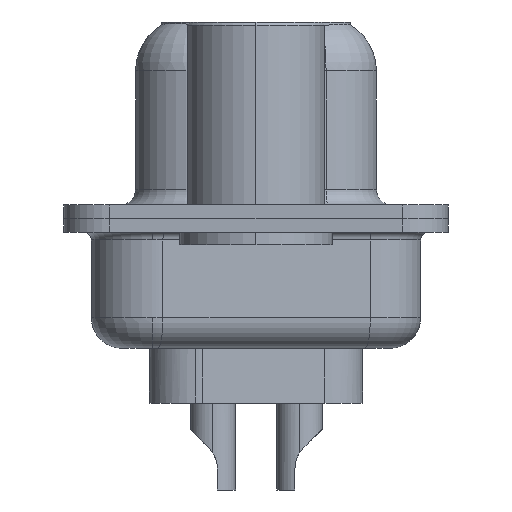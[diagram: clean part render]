
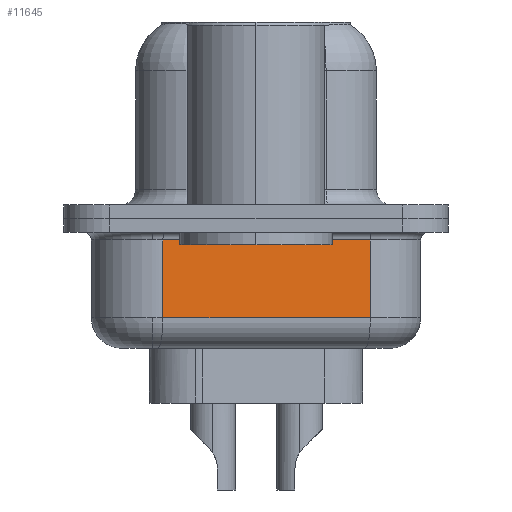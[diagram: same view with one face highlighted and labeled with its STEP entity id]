
A CAD part, left-side view. The second image highlights one B-rep face of the part: STEP entity #11645.
In plain terms, the highlighted planar face has unit normal (-0.985, -0.174, 0).
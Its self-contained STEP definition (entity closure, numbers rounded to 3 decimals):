
#163 = VECTOR ( 'NONE', #10738, 1000. ) ;
#1289 = AXIS2_PLACEMENT_3D ( 'NONE', #15558, #20677, #1568 ) ;
#1568 = DIRECTION ( 'NONE',  ( -0.174, 0.985, 0. ) ) ;
#2050 = DIRECTION ( 'NONE',  ( 0.174, -0.985, 0. ) ) ;
#2419 = EDGE_LOOP ( 'NONE', ( #8720, #7108, #7721, #17372 ) ) ;
#3175 = VERTEX_POINT ( 'NONE', #18210 ) ;
#3624 = DIRECTION ( 'NONE',  ( -0.174, 0.985, 0. ) ) ;
#3971 = CARTESIAN_POINT ( 'NONE',  ( 2.89, 3.053, -0.7 ) ) ;
#6151 = LINE ( 'NONE', #7959, #13923 ) ;
#7108 = ORIENTED_EDGE ( 'NONE', *, *, #14911, .T. ) ;
#7721 = ORIENTED_EDGE ( 'NONE', *, *, #13287, .T. ) ;
#7959 = CARTESIAN_POINT ( 'NONE',  ( 4.089, -3.747, -4.25 ) ) ;
#8642 = VECTOR ( 'NONE', #3624, 1000. ) ;
#8701 = FACE_OUTER_BOUND ( 'NONE', #2419, .T. ) ;
#8720 = ORIENTED_EDGE ( 'NONE', *, *, #21592, .F. ) ;
#10217 = VERTEX_POINT ( 'NONE', #20018 ) ;
#10555 = CARTESIAN_POINT ( 'NONE',  ( 2.89, 3.053, -3.25 ) ) ;
#10738 = DIRECTION ( 'NONE',  ( 0., 0., 1. ) ) ;
#10793 = LINE ( 'NONE', #10555, #12179 ) ;
#11147 = CARTESIAN_POINT ( 'NONE',  ( 2.89, 3.053, -3.25 ) ) ;
#11645 = ADVANCED_FACE ( 'NONE', ( #8701 ), #16831, .F. ) ;
#12179 = VECTOR ( 'NONE', #2050, 1000. ) ;
#12609 = CARTESIAN_POINT ( 'NONE',  ( 2.89, 3.053, -0.7 ) ) ;
#12738 = VERTEX_POINT ( 'NONE', #12609 ) ;
#12853 = LINE ( 'NONE', #19764, #163 ) ;
#13287 = EDGE_CURVE ( 'NONE', #10217, #3175, #6151, .T. ) ;
#13923 = VECTOR ( 'NONE', #14481, 1000. ) ;
#14481 = DIRECTION ( 'NONE',  ( 0., 0., 1. ) ) ;
#14911 = EDGE_CURVE ( 'NONE', #15714, #10217, #10793, .T. ) ;
#15558 = CARTESIAN_POINT ( 'NONE',  ( 2.89, 3.053, -4.25 ) ) ;
#15714 = VERTEX_POINT ( 'NONE', #11147 ) ;
#16729 = EDGE_CURVE ( 'NONE', #3175, #12738, #20935, .T. ) ;
#16831 = PLANE ( 'NONE',  #1289 ) ;
#17372 = ORIENTED_EDGE ( 'NONE', *, *, #16729, .T. ) ;
#18210 = CARTESIAN_POINT ( 'NONE',  ( 4.089, -3.747, -0.7 ) ) ;
#19764 = CARTESIAN_POINT ( 'NONE',  ( 2.89, 3.053, -4.25 ) ) ;
#20018 = CARTESIAN_POINT ( 'NONE',  ( 4.089, -3.747, -3.25 ) ) ;
#20677 = DIRECTION ( 'NONE',  ( 0.985, 0.174, 0. ) ) ;
#20935 = LINE ( 'NONE', #3971, #8642 ) ;
#21592 = EDGE_CURVE ( 'NONE', #15714, #12738, #12853, .T. ) ;
